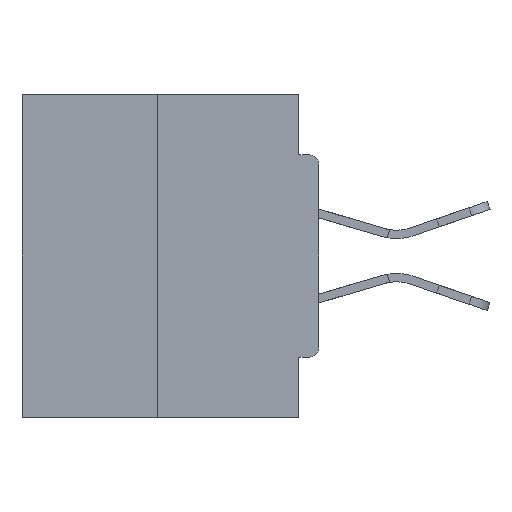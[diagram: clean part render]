
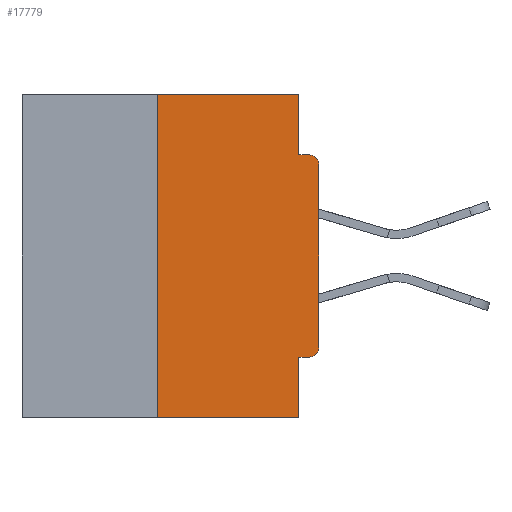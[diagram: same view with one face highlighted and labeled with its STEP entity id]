
A CAD part, left-side view. The second image highlights one B-rep face of the part: STEP entity #17779.
In plain terms, the highlighted planar face has unit normal (-1, 0, 0).
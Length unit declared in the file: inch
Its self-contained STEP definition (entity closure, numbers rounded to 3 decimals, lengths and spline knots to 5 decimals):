
#203 = EDGE_CURVE ( 'NONE', #33621, #34187, #19191, .T. ) ;
#600 = VERTEX_POINT ( 'NONE', #21766 ) ;
#638 = CARTESIAN_POINT ( 'NONE',  ( 0., 0.015, -0.0935 ) ) ;
#897 = VERTEX_POINT ( 'NONE', #20939 ) ;
#1547 = CARTESIAN_POINT ( 'NONE',  ( 0., 0.031, 0. ) ) ;
#1885 = DIRECTION ( 'NONE',  ( 0., 1., 0. ) ) ;
#2212 = LINE ( 'NONE', #11895, #24317 ) ;
#2282 = EDGE_CURVE ( 'NONE', #600, #16715, #2212, .T. ) ;
#2283 = ORIENTED_EDGE ( 'NONE', *, *, #36689, .F. ) ;
#2352 = VECTOR ( 'NONE', #13230, 39.37008 ) ;
#2790 = VECTOR ( 'NONE', #13345, 39.37008 ) ;
#2904 = ORIENTED_EDGE ( 'NONE', *, *, #14159, .T. ) ;
#3387 = CARTESIAN_POINT ( 'NONE',  ( 0., 0.015, -0.1085 ) ) ;
#3663 = DIRECTION ( 'NONE',  ( 0., 0., -1. ) ) ;
#3807 = CARTESIAN_POINT ( 'NONE',  ( 0., 0., -0.1085 ) ) ;
#4694 = CARTESIAN_POINT ( 'NONE',  ( 0., 0., -0.4065 ) ) ;
#4856 = AXIS2_PLACEMENT_3D ( 'NONE', #3387, #27735, #3663 ) ;
#5220 = VECTOR ( 'NONE', #12529, 39.37008 ) ;
#5663 = LINE ( 'NONE', #31908, #2790 ) ;
#5942 = ORIENTED_EDGE ( 'NONE', *, *, #35979, .F. ) ;
#5978 = CIRCLE ( 'NONE', #4856, 0.015 ) ;
#7324 = EDGE_CURVE ( 'NONE', #897, #7755, #12877, .T. ) ;
#7585 = VECTOR ( 'NONE', #1885, 39.37008 ) ;
#7755 = VERTEX_POINT ( 'NONE', #25614 ) ;
#7866 = EDGE_CURVE ( 'NONE', #897, #600, #18608, .T. ) ;
#7914 = PLANE ( 'NONE',  #35610 ) ;
#9314 = CARTESIAN_POINT ( 'NONE',  ( 0., 0., -0.0935 ) ) ;
#9337 = LINE ( 'NONE', #37182, #28093 ) ;
#9996 = LINE ( 'NONE', #9314, #5220 ) ;
#10510 = VECTOR ( 'NONE', #22633, 39.37008 ) ;
#11293 = DIRECTION ( 'NONE',  ( 0., -1., 0. ) ) ;
#11399 = CARTESIAN_POINT ( 'NONE',  ( 0., 0.031, -0.0935 ) ) ;
#11502 = CARTESIAN_POINT ( 'NONE',  ( 0., 0.031, 0. ) ) ;
#11895 = CARTESIAN_POINT ( 'NONE',  ( 0., 0., 0. ) ) ;
#12529 = DIRECTION ( 'NONE',  ( 0., -1., 0. ) ) ;
#12877 = LINE ( 'NONE', #4694, #7585 ) ;
#13230 = DIRECTION ( 'NONE',  ( 0., 0., -1. ) ) ;
#13345 = DIRECTION ( 'NONE',  ( 0., 0., -1. ) ) ;
#13385 = VERTEX_POINT ( 'NONE', #11502 ) ;
#13558 = EDGE_CURVE ( 'NONE', #33621, #26795, #9337, .T. ) ;
#13688 = CARTESIAN_POINT ( 'NONE',  ( 0., 0.031, -0.5 ) ) ;
#14159 = EDGE_CURVE ( 'NONE', #16715, #14789, #5978, .T. ) ;
#14569 = DIRECTION ( 'NONE',  ( 0., 0., -1. ) ) ;
#14570 = ORIENTED_EDGE ( 'NONE', *, *, #203, .F. ) ;
#14789 = VERTEX_POINT ( 'NONE', #638 ) ;
#15258 = ORIENTED_EDGE ( 'NONE', *, *, #22932, .F. ) ;
#16715 = VERTEX_POINT ( 'NONE', #3807 ) ;
#17751 = ORIENTED_EDGE ( 'NONE', *, *, #2282, .T. ) ;
#17779 = ADVANCED_FACE ( 'NONE', ( #19469 ), #7914, .F. ) ;
#18608 = CIRCLE ( 'NONE', #31728, 0.015 ) ;
#19191 = LINE ( 'NONE', #19406, #10510 ) ;
#19257 = DIRECTION ( 'NONE',  ( 0., -1., 0. ) ) ;
#19406 = CARTESIAN_POINT ( 'NONE',  ( 0., 0.25, 0. ) ) ;
#19469 = FACE_OUTER_BOUND ( 'NONE', #25556, .T. ) ;
#20360 = CARTESIAN_POINT ( 'NONE',  ( 0., 0.015, -0.3915 ) ) ;
#20699 = CARTESIAN_POINT ( 'NONE',  ( 0., 0.46, 0. ) ) ;
#20939 = CARTESIAN_POINT ( 'NONE',  ( 0., 0.015, -0.4065 ) ) ;
#21766 = CARTESIAN_POINT ( 'NONE',  ( 0., 0., -0.3915 ) ) ;
#21977 = VERTEX_POINT ( 'NONE', #11399 ) ;
#22633 = DIRECTION ( 'NONE',  ( 0., 0., 1. ) ) ;
#22932 = EDGE_CURVE ( 'NONE', #7755, #26795, #5663, .T. ) ;
#23481 = DIRECTION ( 'NONE',  ( -1., 0., 0. ) ) ;
#24317 = VECTOR ( 'NONE', #30604, 39.37008 ) ;
#25009 = ORIENTED_EDGE ( 'NONE', *, *, #7324, .F. ) ;
#25472 = CARTESIAN_POINT ( 'NONE',  ( 0., 0.25, -0.5 ) ) ;
#25556 = EDGE_LOOP ( 'NONE', ( #2283, #14570, #34819, #15258, #25009, #38334, #17751, #2904, #34115, #5942 ) ) ;
#25614 = CARTESIAN_POINT ( 'NONE',  ( 0., 0.031, -0.4065 ) ) ;
#26087 = CARTESIAN_POINT ( 'NONE',  ( 0., 0.46, 0. ) ) ;
#26350 = VECTOR ( 'NONE', #11293, 39.37008 ) ;
#26795 = VERTEX_POINT ( 'NONE', #13688 ) ;
#27735 = DIRECTION ( 'NONE',  ( -1., 0., 0. ) ) ;
#28093 = VECTOR ( 'NONE', #19257, 39.37008 ) ;
#28140 = CARTESIAN_POINT ( 'NONE',  ( 0., 0.25, 0. ) ) ;
#29183 = DIRECTION ( 'NONE',  ( 1., 0., 0. ) ) ;
#30604 = DIRECTION ( 'NONE',  ( 0., 0., 1. ) ) ;
#31728 = AXIS2_PLACEMENT_3D ( 'NONE', #20360, #23481, #14569 ) ;
#31908 = CARTESIAN_POINT ( 'NONE',  ( 0., 0.031, -0.5 ) ) ;
#33146 = LINE ( 'NONE', #1547, #2352 ) ;
#33621 = VERTEX_POINT ( 'NONE', #25472 ) ;
#34115 = ORIENTED_EDGE ( 'NONE', *, *, #36209, .F. ) ;
#34187 = VERTEX_POINT ( 'NONE', #28140 ) ;
#34819 = ORIENTED_EDGE ( 'NONE', *, *, #13558, .T. ) ;
#35474 = LINE ( 'NONE', #20699, #26350 ) ;
#35610 = AXIS2_PLACEMENT_3D ( 'NONE', #26087, #29183, #38433 ) ;
#35979 = EDGE_CURVE ( 'NONE', #13385, #21977, #33146, .T. ) ;
#36209 = EDGE_CURVE ( 'NONE', #21977, #14789, #9996, .T. ) ;
#36689 = EDGE_CURVE ( 'NONE', #34187, #13385, #35474, .T. ) ;
#37182 = CARTESIAN_POINT ( 'NONE',  ( 0., 0.46, -0.5 ) ) ;
#38334 = ORIENTED_EDGE ( 'NONE', *, *, #7866, .T. ) ;
#38433 = DIRECTION ( 'NONE',  ( 0., 0., -1. ) ) ;
